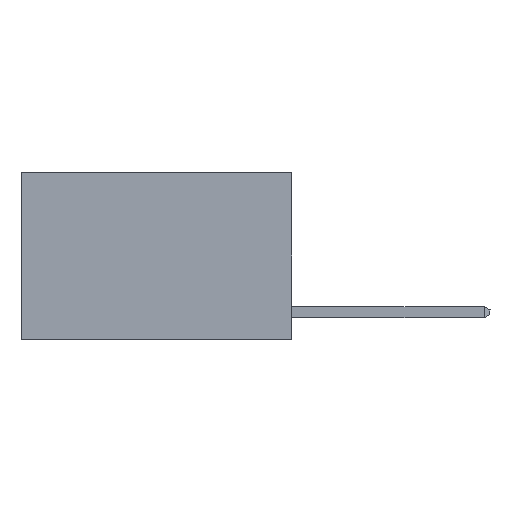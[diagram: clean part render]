
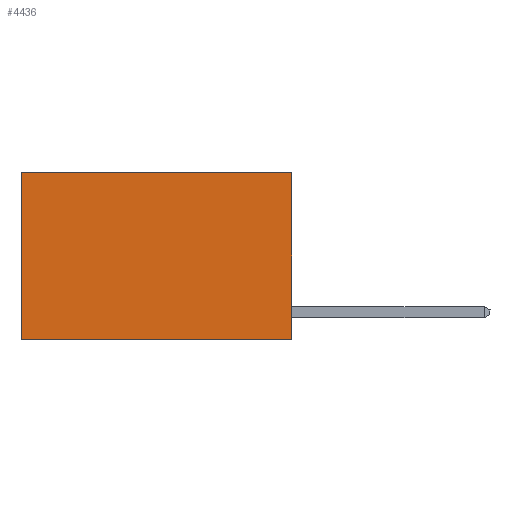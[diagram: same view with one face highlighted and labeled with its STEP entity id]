
A CAD part, left-side view. The second image highlights one B-rep face of the part: STEP entity #4436.
In plain terms, the highlighted planar face has unit normal (-1, 0, 0).
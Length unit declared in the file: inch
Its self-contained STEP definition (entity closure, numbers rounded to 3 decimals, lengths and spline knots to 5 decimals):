
#703 = DIRECTION ( 'NONE',  ( 0., 0., -1. ) ) ;
#1256 = EDGE_CURVE ( 'NONE', #4315, #7328, #6089, .T. ) ;
#2025 = LINE ( 'NONE', #21579, #21846 ) ;
#3067 = LINE ( 'NONE', #17374, #14034 ) ;
#3811 = ORIENTED_EDGE ( 'NONE', *, *, #23652, .T. ) ;
#4315 = VERTEX_POINT ( 'NONE', #21042 ) ;
#4331 = EDGE_CURVE ( 'NONE', #22378, #4315, #3067, .T. ) ;
#4436 = ADVANCED_FACE ( 'NONE', ( #9815 ), #8619, .F. ) ;
#5083 = VECTOR ( 'NONE', #18117, 39.37008 ) ;
#5901 = DIRECTION ( 'NONE',  ( 0., 0., -1. ) ) ;
#6089 = LINE ( 'NONE', #8205, #11235 ) ;
#7328 = VERTEX_POINT ( 'NONE', #8043 ) ;
#8043 = CARTESIAN_POINT ( 'NONE',  ( 0.2625, 0.6, -0.37 ) ) ;
#8205 = CARTESIAN_POINT ( 'NONE',  ( 0.2625, 0., -0.37 ) ) ;
#8361 = DIRECTION ( 'NONE',  ( 0., 1., 0. ) ) ;
#8619 = PLANE ( 'NONE',  #18243 ) ;
#9815 = FACE_OUTER_BOUND ( 'NONE', #18946, .T. ) ;
#9886 = EDGE_CURVE ( 'NONE', #22378, #18559, #2025, .T. ) ;
#10251 = ORIENTED_EDGE ( 'NONE', *, *, #4331, .F. ) ;
#11235 = VECTOR ( 'NONE', #13079, 39.37008 ) ;
#12424 = CARTESIAN_POINT ( 'NONE',  ( 0.2625, 0.6, 0. ) ) ;
#12495 = DIRECTION ( 'NONE',  ( 1., 0., 0. ) ) ;
#13079 = DIRECTION ( 'NONE',  ( 0., 1., 0. ) ) ;
#13757 = CARTESIAN_POINT ( 'NONE',  ( 0.2625, 0., 0. ) ) ;
#14034 = VECTOR ( 'NONE', #5901, 39.37008 ) ;
#15309 = LINE ( 'NONE', #12424, #5083 ) ;
#17374 = CARTESIAN_POINT ( 'NONE',  ( 0.2625, 0., 0. ) ) ;
#18111 = CARTESIAN_POINT ( 'NONE',  ( 0.2625, 0., 0. ) ) ;
#18117 = DIRECTION ( 'NONE',  ( 0., 0., -1. ) ) ;
#18243 = AXIS2_PLACEMENT_3D ( 'NONE', #18111, #12495, #703 ) ;
#18559 = VERTEX_POINT ( 'NONE', #22043 ) ;
#18946 = EDGE_LOOP ( 'NONE', ( #3811, #24625, #10251, #20317 ) ) ;
#20317 = ORIENTED_EDGE ( 'NONE', *, *, #9886, .T. ) ;
#21042 = CARTESIAN_POINT ( 'NONE',  ( 0.2625, 0., -0.37 ) ) ;
#21579 = CARTESIAN_POINT ( 'NONE',  ( 0.2625, 0., 0. ) ) ;
#21846 = VECTOR ( 'NONE', #8361, 39.37008 ) ;
#22043 = CARTESIAN_POINT ( 'NONE',  ( 0.2625, 0.6, 0. ) ) ;
#22378 = VERTEX_POINT ( 'NONE', #13757 ) ;
#23652 = EDGE_CURVE ( 'NONE', #18559, #7328, #15309, .T. ) ;
#24625 = ORIENTED_EDGE ( 'NONE', *, *, #1256, .F. ) ;
